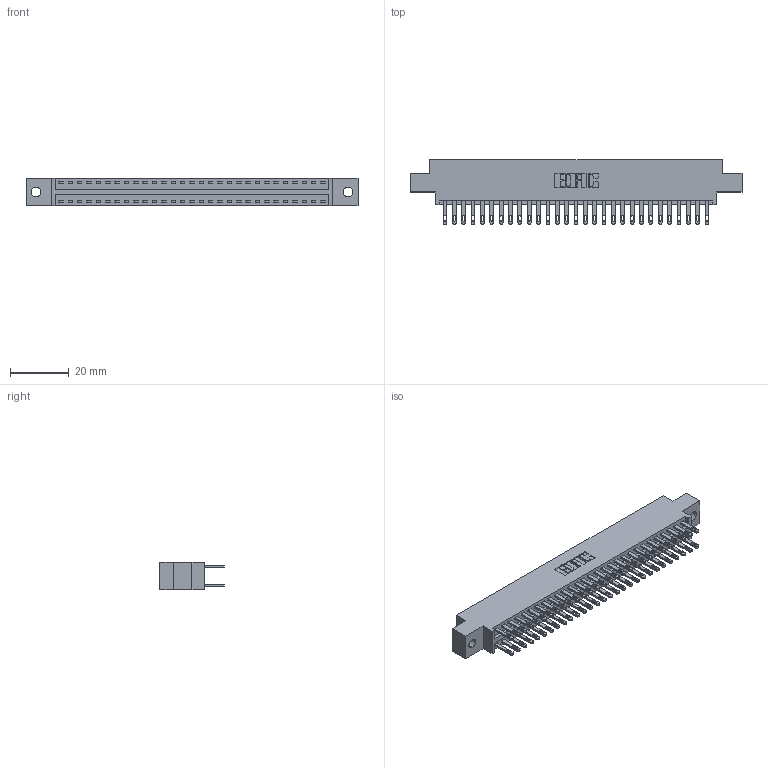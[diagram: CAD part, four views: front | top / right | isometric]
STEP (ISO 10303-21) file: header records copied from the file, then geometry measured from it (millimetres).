
FILE_DESCRIPTION (( 'STEP AP203' ), '1' );
FILE_NAME ('346-058-500-802.STEP', '2018-08-28T03:36:43', ( '' ), ( '' ), 'SwSTEP 2.0', 'SolidWorks 2016', '' );
FILE_SCHEMA (( 'CONFIG_CONTROL_DESIGN' ));
Length unit declared in the file: inch
Products named in the file (3): 346 Part_0.170 Offset - 0.128 Dia; 345-292-001_345-293-100; 346-058-500-802
Assembly tree (59 placements, depth 2):
  346-058-500-802
    346 Part_0.170 Offset - 0.128 Dia
    345-292-001_345-293-100  x58
Bounding box: 112.65 x 21.84 x 9.4 mm (x, y, z)
Volume: 10869.7 mm3; surface area: 15254.2 mm2
Topology: 59 solids, 59 shells, 2910 faces, 8867 edges, 5910 vertices
Faces by surface type: plane 1762, cylinder 1148
Entity records: 20741 total; most frequent: CARTESIAN_POINT 3436, ORIENTED_EDGE 3370, DIRECTION 3081, EDGE_CURVE 1685, VECTOR 1433, LINE 1433, VERTEX_POINT 1122, AXIS2_PLACEMENT_3D 824
